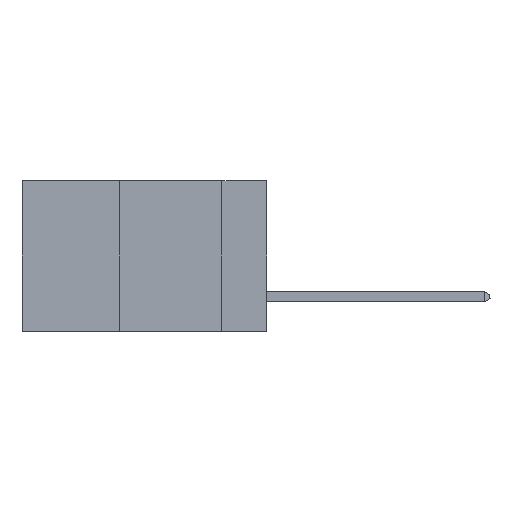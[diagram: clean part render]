
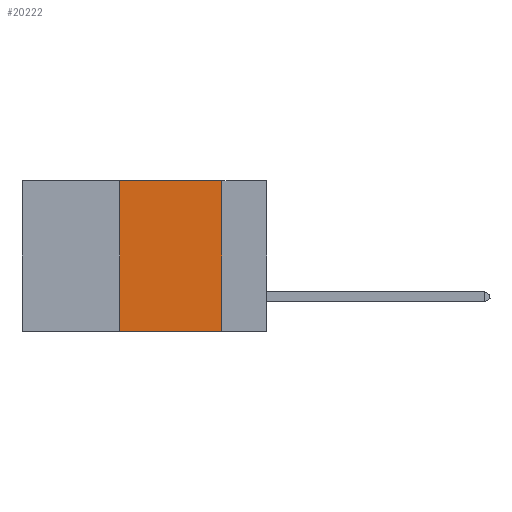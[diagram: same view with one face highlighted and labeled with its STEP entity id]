
A CAD part, left-side view. The second image highlights one B-rep face of the part: STEP entity #20222.
In plain terms, the highlighted planar face has unit normal (-1, 0, 0).
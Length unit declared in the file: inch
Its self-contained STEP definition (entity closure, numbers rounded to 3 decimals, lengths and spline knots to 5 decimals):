
#307 = PLANE ( 'NONE',  #4102 ) ;
#1606 = EDGE_CURVE ( 'NONE', #1948, #5701, #7805, .T. ) ;
#1863 = CARTESIAN_POINT ( 'NONE',  ( 0., 0.6, 0. ) ) ;
#1948 = VERTEX_POINT ( 'NONE', #23725 ) ;
#2062 = LINE ( 'NONE', #13339, #10768 ) ;
#2539 = EDGE_LOOP ( 'NONE', ( #25230, #19557, #22185, #7694 ) ) ;
#2759 = CARTESIAN_POINT ( 'NONE',  ( 0., 0.6, -0.37 ) ) ;
#2954 = DIRECTION ( 'NONE',  ( 0., 0., -1. ) ) ;
#4102 = AXIS2_PLACEMENT_3D ( 'NONE', #1863, #17744, #2954 ) ;
#4229 = VECTOR ( 'NONE', #10526, 39.37008 ) ;
#4808 = CARTESIAN_POINT ( 'NONE',  ( 0., 0.36, 0. ) ) ;
#5358 = VERTEX_POINT ( 'NONE', #25395 ) ;
#5701 = VERTEX_POINT ( 'NONE', #20706 ) ;
#6796 = DIRECTION ( 'NONE',  ( 0., 0., 1. ) ) ;
#7694 = ORIENTED_EDGE ( 'NONE', *, *, #19034, .T. ) ;
#7805 = LINE ( 'NONE', #4808, #22945 ) ;
#7991 = LINE ( 'NONE', #2759, #4229 ) ;
#10526 = DIRECTION ( 'NONE',  ( 0., -1., 0. ) ) ;
#10768 = VECTOR ( 'NONE', #25328, 39.37008 ) ;
#13339 = CARTESIAN_POINT ( 'NONE',  ( 0., 0.11, 0. ) ) ;
#15609 = EDGE_CURVE ( 'NONE', #5358, #22481, #2062, .T. ) ;
#16095 = CARTESIAN_POINT ( 'NONE',  ( 0., 0.6, 0. ) ) ;
#16582 = LINE ( 'NONE', #16095, #20242 ) ;
#17676 = EDGE_CURVE ( 'NONE', #5701, #5358, #16582, .T. ) ;
#17744 = DIRECTION ( 'NONE',  ( 1., 0., 0. ) ) ;
#19034 = EDGE_CURVE ( 'NONE', #1948, #22481, #7991, .T. ) ;
#19230 = CARTESIAN_POINT ( 'NONE',  ( 0., 0.11, -0.37 ) ) ;
#19557 = ORIENTED_EDGE ( 'NONE', *, *, #17676, .F. ) ;
#20006 = DIRECTION ( 'NONE',  ( 0., -1., 0. ) ) ;
#20222 = ADVANCED_FACE ( 'NONE', ( #21817 ), #307, .F. ) ;
#20242 = VECTOR ( 'NONE', #20006, 39.37008 ) ;
#20706 = CARTESIAN_POINT ( 'NONE',  ( 0., 0.36, 0. ) ) ;
#21817 = FACE_OUTER_BOUND ( 'NONE', #2539, .T. ) ;
#22185 = ORIENTED_EDGE ( 'NONE', *, *, #1606, .F. ) ;
#22481 = VERTEX_POINT ( 'NONE', #19230 ) ;
#22945 = VECTOR ( 'NONE', #6796, 39.37008 ) ;
#23725 = CARTESIAN_POINT ( 'NONE',  ( 0., 0.36, -0.37 ) ) ;
#25230 = ORIENTED_EDGE ( 'NONE', *, *, #15609, .F. ) ;
#25328 = DIRECTION ( 'NONE',  ( 0., 0., -1. ) ) ;
#25395 = CARTESIAN_POINT ( 'NONE',  ( 0., 0.11, 0. ) ) ;
